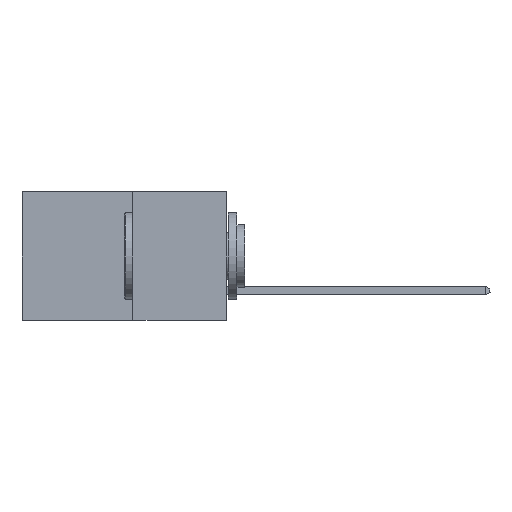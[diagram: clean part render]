
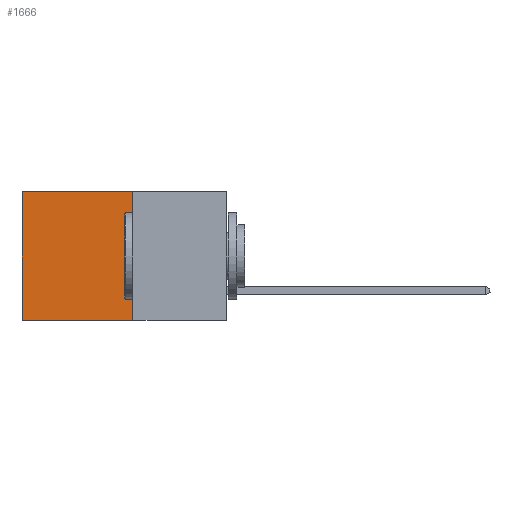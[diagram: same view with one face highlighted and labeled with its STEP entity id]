
A CAD part, left-side view. The second image highlights one B-rep face of the part: STEP entity #1666.
In plain terms, the highlighted planar face has unit normal (-1, 0, 0).
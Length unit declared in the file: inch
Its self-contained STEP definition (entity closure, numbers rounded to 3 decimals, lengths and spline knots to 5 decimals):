
#216 = LINE ( 'NONE', #13906, #13036 ) ;
#737 = EDGE_CURVE ( 'NONE', #16157, #7799, #4264, .T. ) ;
#1026 = ORIENTED_EDGE ( 'NONE', *, *, #11877, .F. ) ;
#1666 = ADVANCED_FACE ( 'NONE', ( #20224 ), #8743, .F. ) ;
#1862 = ORIENTED_EDGE ( 'NONE', *, *, #20645, .F. ) ;
#3259 = CARTESIAN_POINT ( 'NONE',  ( 0.277, 0.27, 0. ) ) ;
#4264 = LINE ( 'NONE', #13098, #12073 ) ;
#5187 = DIRECTION ( 'NONE',  ( 0., 0., -1. ) ) ;
#7219 = EDGE_LOOP ( 'NONE', ( #13812, #1862, #1026, #17224 ) ) ;
#7799 = VERTEX_POINT ( 'NONE', #12963 ) ;
#8563 = CARTESIAN_POINT ( 'NONE',  ( 0.277, 0.27, -0.37 ) ) ;
#8743 = PLANE ( 'NONE',  #21001 ) ;
#9991 = CARTESIAN_POINT ( 'NONE',  ( 0.277, 0.27, 0. ) ) ;
#11506 = CARTESIAN_POINT ( 'NONE',  ( 0.277, 0.27, -0.37 ) ) ;
#11877 = EDGE_CURVE ( 'NONE', #20431, #19157, #20335, .T. ) ;
#12073 = VECTOR ( 'NONE', #14987, 39.37008 ) ;
#12210 = CARTESIAN_POINT ( 'NONE',  ( 0.277, 0.59, 0. ) ) ;
#12963 = CARTESIAN_POINT ( 'NONE',  ( 0.277, 0.59, -0.37 ) ) ;
#13036 = VECTOR ( 'NONE', #15577, 39.37008 ) ;
#13098 = CARTESIAN_POINT ( 'NONE',  ( 0.277, 0.59, -0.37 ) ) ;
#13812 = ORIENTED_EDGE ( 'NONE', *, *, #737, .T. ) ;
#13906 = CARTESIAN_POINT ( 'NONE',  ( 0.277, 0.27, -0.37 ) ) ;
#14741 = VECTOR ( 'NONE', #16558, 39.37008 ) ;
#14987 = DIRECTION ( 'NONE',  ( 0., 0., -1. ) ) ;
#15254 = LINE ( 'NONE', #3259, #14741 ) ;
#15577 = DIRECTION ( 'NONE',  ( 0., 1., 0. ) ) ;
#16045 = VECTOR ( 'NONE', #5187, 39.37008 ) ;
#16157 = VERTEX_POINT ( 'NONE', #12210 ) ;
#16558 = DIRECTION ( 'NONE',  ( 0., 1., 0. ) ) ;
#17224 = ORIENTED_EDGE ( 'NONE', *, *, #19774, .T. ) ;
#17996 = CARTESIAN_POINT ( 'NONE',  ( 0.277, 0.27, -0.37 ) ) ;
#18072 = DIRECTION ( 'NONE',  ( 1., 0., 0. ) ) ;
#18275 = DIRECTION ( 'NONE',  ( 0., 0., -1. ) ) ;
#19157 = VERTEX_POINT ( 'NONE', #11506 ) ;
#19774 = EDGE_CURVE ( 'NONE', #20431, #16157, #15254, .T. ) ;
#20224 = FACE_OUTER_BOUND ( 'NONE', #7219, .T. ) ;
#20335 = LINE ( 'NONE', #8563, #16045 ) ;
#20431 = VERTEX_POINT ( 'NONE', #9991 ) ;
#20645 = EDGE_CURVE ( 'NONE', #19157, #7799, #216, .T. ) ;
#21001 = AXIS2_PLACEMENT_3D ( 'NONE', #17996, #18072, #18275 ) ;
